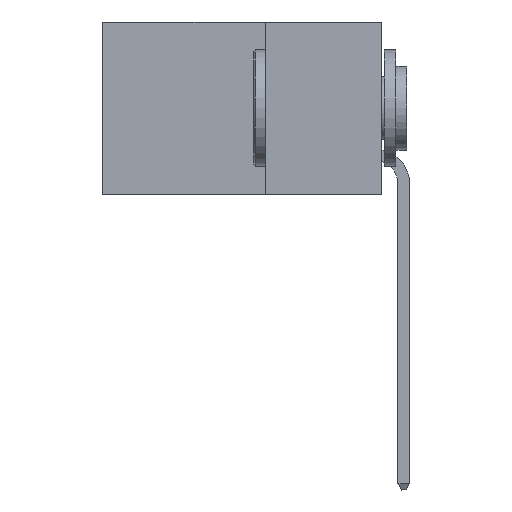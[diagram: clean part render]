
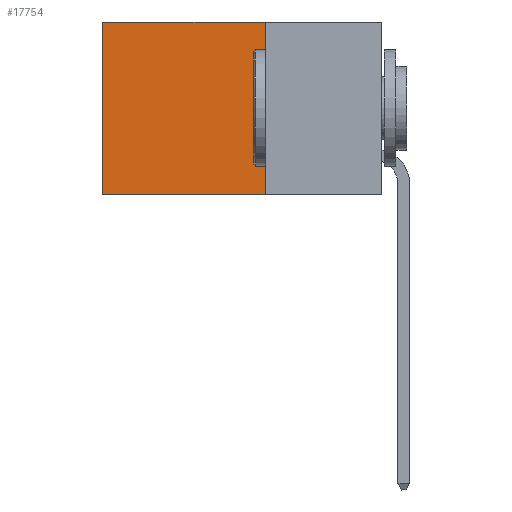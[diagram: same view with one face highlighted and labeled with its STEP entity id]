
A CAD part, left-side view. The second image highlights one B-rep face of the part: STEP entity #17754.
In plain terms, the highlighted planar face has unit normal (-1, 0, 0).
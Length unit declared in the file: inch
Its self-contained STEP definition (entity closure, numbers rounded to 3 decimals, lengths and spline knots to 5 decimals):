
#762 = ORIENTED_EDGE ( 'NONE', *, *, #11894, .F. ) ;
#2042 = CARTESIAN_POINT ( 'NONE',  ( 0.2875, 0.25, 0. ) ) ;
#2057 = PLANE ( 'NONE',  #21537 ) ;
#2131 = VECTOR ( 'NONE', #9841, 39.37008 ) ;
#2330 = CARTESIAN_POINT ( 'NONE',  ( 0.2875, 0.6, 0. ) ) ;
#3856 = CARTESIAN_POINT ( 'NONE',  ( 0.2875, 0.25, 0. ) ) ;
#6514 = LINE ( 'NONE', #8333, #6794 ) ;
#6794 = VECTOR ( 'NONE', #13234, 39.37008 ) ;
#8333 = CARTESIAN_POINT ( 'NONE',  ( 0.2875, 0.25, -0.37 ) ) ;
#9208 = DIRECTION ( 'NONE',  ( 0., 0., -1. ) ) ;
#9411 = DIRECTION ( 'NONE',  ( 0., 0., -1. ) ) ;
#9841 = DIRECTION ( 'NONE',  ( 0., 0., -1. ) ) ;
#10922 = EDGE_CURVE ( 'NONE', #22343, #21463, #13377, .T. ) ;
#11025 = LINE ( 'NONE', #2042, #11589 ) ;
#11589 = VECTOR ( 'NONE', #9411, 39.37008 ) ;
#11894 = EDGE_CURVE ( 'NONE', #22343, #14776, #11025, .T. ) ;
#12041 = EDGE_LOOP ( 'NONE', ( #15347, #17609, #762, #21319 ) ) ;
#13234 = DIRECTION ( 'NONE',  ( 0., 1., 0. ) ) ;
#13269 = CARTESIAN_POINT ( 'NONE',  ( 0.2875, 0.6, -0.37 ) ) ;
#13377 = LINE ( 'NONE', #14024, #16528 ) ;
#14024 = CARTESIAN_POINT ( 'NONE',  ( 0.2875, 0.25, 0. ) ) ;
#14776 = VERTEX_POINT ( 'NONE', #18584 ) ;
#14809 = FACE_OUTER_BOUND ( 'NONE', #12041, .T. ) ;
#15347 = ORIENTED_EDGE ( 'NONE', *, *, #19756, .T. ) ;
#16528 = VECTOR ( 'NONE', #21389, 39.37008 ) ;
#16531 = VERTEX_POINT ( 'NONE', #13269 ) ;
#16641 = CARTESIAN_POINT ( 'NONE',  ( 0.2875, 0.6, 0. ) ) ;
#17609 = ORIENTED_EDGE ( 'NONE', *, *, #18224, .F. ) ;
#17754 = ADVANCED_FACE ( 'NONE', ( #14809 ), #2057, .F. ) ;
#18224 = EDGE_CURVE ( 'NONE', #14776, #16531, #6514, .T. ) ;
#18290 = CARTESIAN_POINT ( 'NONE',  ( 0.2875, 0.25, 0. ) ) ;
#18584 = CARTESIAN_POINT ( 'NONE',  ( 0.2875, 0.25, -0.37 ) ) ;
#19756 = EDGE_CURVE ( 'NONE', #21463, #16531, #22428, .T. ) ;
#21319 = ORIENTED_EDGE ( 'NONE', *, *, #10922, .T. ) ;
#21389 = DIRECTION ( 'NONE',  ( 0., 1., 0. ) ) ;
#21463 = VERTEX_POINT ( 'NONE', #16641 ) ;
#21537 = AXIS2_PLACEMENT_3D ( 'NONE', #18290, #23686, #9208 ) ;
#22343 = VERTEX_POINT ( 'NONE', #3856 ) ;
#22428 = LINE ( 'NONE', #2330, #2131 ) ;
#23686 = DIRECTION ( 'NONE',  ( 1., 0., 0. ) ) ;
